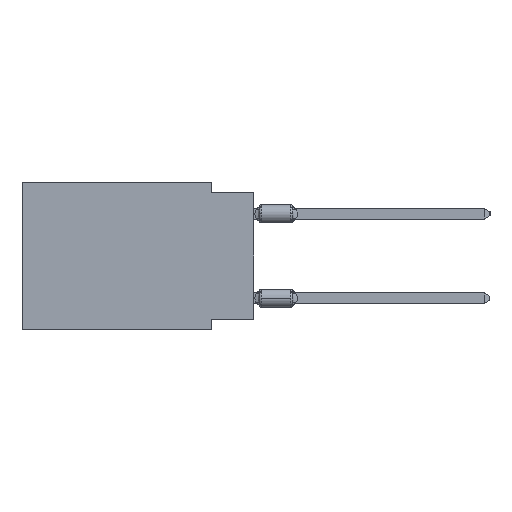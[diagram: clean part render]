
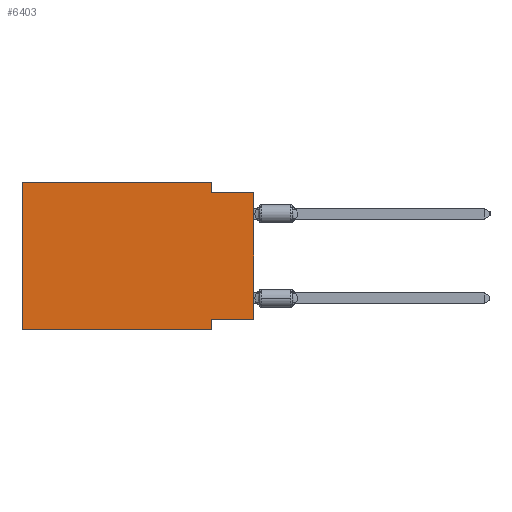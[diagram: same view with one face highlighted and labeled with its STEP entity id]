
A CAD part, left-side view. The second image highlights one B-rep face of the part: STEP entity #6403.
In plain terms, the highlighted planar face has unit normal (-1, 0, 0).
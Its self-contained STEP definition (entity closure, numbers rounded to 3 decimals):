
#68 = LINE ( 'NONE', #17183, #25738 ) ;
#137 = DIRECTION ( 'NONE',  ( 0., 0., -1. ) ) ;
#193 = LINE ( 'NONE', #27516, #31209 ) ;
#638 = ORIENTED_EDGE ( 'NONE', *, *, #22983, .F. ) ;
#1011 = CARTESIAN_POINT ( 'NONE',  ( 0., 2.54, -8.89 ) ) ;
#2461 = LINE ( 'NONE', #22533, #9462 ) ;
#2491 = CARTESIAN_POINT ( 'NONE',  ( 0., 2.54, -8.255 ) ) ;
#2608 = VECTOR ( 'NONE', #14017, 1000. ) ;
#2936 = EDGE_CURVE ( 'NONE', #5706, #6744, #193, .T. ) ;
#4144 = DIRECTION ( 'NONE',  ( 0., -1., 0. ) ) ;
#4324 = LINE ( 'NONE', #9587, #2608 ) ;
#5706 = VERTEX_POINT ( 'NONE', #18614 ) ;
#6373 = VECTOR ( 'NONE', #28233, 1000. ) ;
#6403 = ADVANCED_FACE ( 'NONE', ( #11799 ), #17900, .F. ) ;
#6507 = ORIENTED_EDGE ( 'NONE', *, *, #14684, .F. ) ;
#6744 = VERTEX_POINT ( 'NONE', #29383 ) ;
#6974 = CARTESIAN_POINT ( 'NONE',  ( 0., 13.97, 0. ) ) ;
#8385 = DIRECTION ( 'NONE',  ( 0., 0., 1. ) ) ;
#8554 = CARTESIAN_POINT ( 'NONE',  ( 0., 13.97, 0. ) ) ;
#9205 = AXIS2_PLACEMENT_3D ( 'NONE', #27939, #30254, #137 ) ;
#9462 = VECTOR ( 'NONE', #31918, 1000. ) ;
#9587 = CARTESIAN_POINT ( 'NONE',  ( 0., 2.54, 0. ) ) ;
#10548 = VERTEX_POINT ( 'NONE', #26063 ) ;
#11777 = CARTESIAN_POINT ( 'NONE',  ( 0., 2.54, 0. ) ) ;
#11799 = FACE_OUTER_BOUND ( 'NONE', #23694, .T. ) ;
#12554 = DIRECTION ( 'NONE',  ( 0., -1., 0. ) ) ;
#12695 = VERTEX_POINT ( 'NONE', #6974 ) ;
#13171 = CARTESIAN_POINT ( 'NONE',  ( 0., 13.97, -8.89 ) ) ;
#13946 = VERTEX_POINT ( 'NONE', #1011 ) ;
#14017 = DIRECTION ( 'NONE',  ( 0., 0., -1. ) ) ;
#14194 = VECTOR ( 'NONE', #8385, 1000. ) ;
#14684 = EDGE_CURVE ( 'NONE', #5706, #20884, #2461, .T. ) ;
#15152 = DIRECTION ( 'NONE',  ( 0., 0., 1. ) ) ;
#15921 = ORIENTED_EDGE ( 'NONE', *, *, #2936, .T. ) ;
#16812 = CARTESIAN_POINT ( 'NONE',  ( 0., 13.97, -8.89 ) ) ;
#17183 = CARTESIAN_POINT ( 'NONE',  ( 0., 13.97, 0. ) ) ;
#17809 = EDGE_CURVE ( 'NONE', #22834, #10548, #4324, .T. ) ;
#17900 = PLANE ( 'NONE',  #9205 ) ;
#17998 = LINE ( 'NONE', #18161, #26794 ) ;
#18087 = VERTEX_POINT ( 'NONE', #13171 ) ;
#18161 = CARTESIAN_POINT ( 'NONE',  ( 0., 0., -0.635 ) ) ;
#18614 = CARTESIAN_POINT ( 'NONE',  ( 0., 0., -8.255 ) ) ;
#20884 = VERTEX_POINT ( 'NONE', #2491 ) ;
#21996 = DIRECTION ( 'NONE',  ( 0., -1., 0. ) ) ;
#22533 = CARTESIAN_POINT ( 'NONE',  ( 0., 0., -8.255 ) ) ;
#22834 = VERTEX_POINT ( 'NONE', #11777 ) ;
#22983 = EDGE_CURVE ( 'NONE', #10548, #6744, #17998, .T. ) ;
#23210 = LINE ( 'NONE', #8554, #14194 ) ;
#23265 = EDGE_CURVE ( 'NONE', #18087, #13946, #26680, .T. ) ;
#23519 = EDGE_CURVE ( 'NONE', #18087, #12695, #23210, .T. ) ;
#23694 = EDGE_LOOP ( 'NONE', ( #15921, #638, #30839, #30788, #26280, #28751, #26284, #6507 ) ) ;
#24179 = VECTOR ( 'NONE', #4144, 1000. ) ;
#25738 = VECTOR ( 'NONE', #12554, 1000. ) ;
#25771 = CARTESIAN_POINT ( 'NONE',  ( 0., 2.54, -8.89 ) ) ;
#26063 = CARTESIAN_POINT ( 'NONE',  ( 0., 2.54, -0.635 ) ) ;
#26280 = ORIENTED_EDGE ( 'NONE', *, *, #23519, .F. ) ;
#26284 = ORIENTED_EDGE ( 'NONE', *, *, #29533, .F. ) ;
#26680 = LINE ( 'NONE', #16812, #24179 ) ;
#26794 = VECTOR ( 'NONE', #21996, 1000. ) ;
#27516 = CARTESIAN_POINT ( 'NONE',  ( 0., 0., 0. ) ) ;
#27939 = CARTESIAN_POINT ( 'NONE',  ( 0., 13.97, 0. ) ) ;
#28233 = DIRECTION ( 'NONE',  ( 0., 0., -1. ) ) ;
#28274 = EDGE_CURVE ( 'NONE', #12695, #22834, #68, .T. ) ;
#28556 = LINE ( 'NONE', #25771, #6373 ) ;
#28751 = ORIENTED_EDGE ( 'NONE', *, *, #23265, .T. ) ;
#29383 = CARTESIAN_POINT ( 'NONE',  ( 0., 0., -0.635 ) ) ;
#29533 = EDGE_CURVE ( 'NONE', #20884, #13946, #28556, .T. ) ;
#30254 = DIRECTION ( 'NONE',  ( 1., 0., 0. ) ) ;
#30788 = ORIENTED_EDGE ( 'NONE', *, *, #28274, .F. ) ;
#30839 = ORIENTED_EDGE ( 'NONE', *, *, #17809, .F. ) ;
#31209 = VECTOR ( 'NONE', #15152, 1000. ) ;
#31918 = DIRECTION ( 'NONE',  ( 0., 1., 0. ) ) ;
